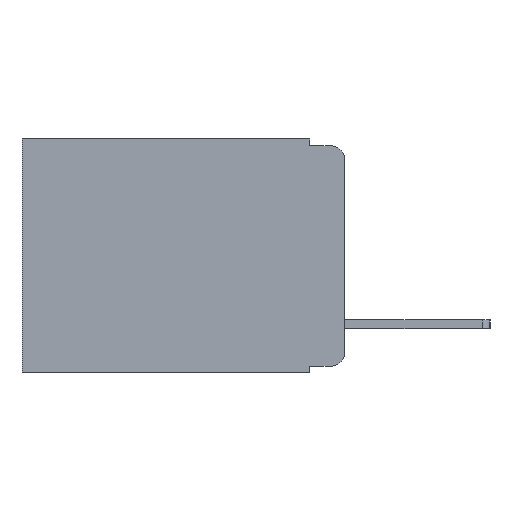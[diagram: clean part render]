
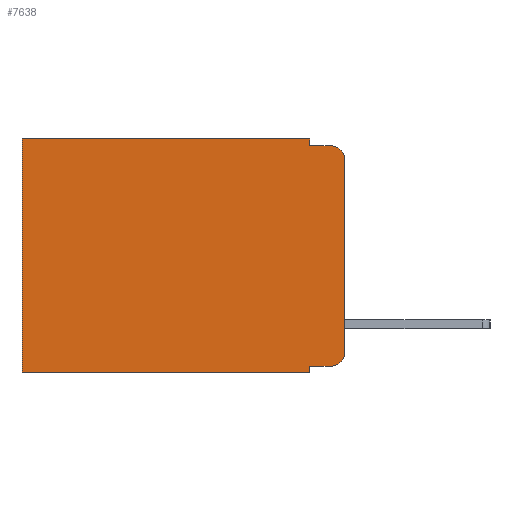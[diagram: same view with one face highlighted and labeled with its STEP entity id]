
A CAD part, left-side view. The second image highlights one B-rep face of the part: STEP entity #7638.
In plain terms, the highlighted planar face has unit normal (-1, 0, 0).
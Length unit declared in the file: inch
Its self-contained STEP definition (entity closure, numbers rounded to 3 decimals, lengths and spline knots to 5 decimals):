
#141 = LINE ( 'NONE', #13781, #4481 ) ;
#309 = DIRECTION ( 'NONE',  ( 0., 1., 0. ) ) ;
#424 = CARTESIAN_POINT ( 'NONE',  ( 0.298, 0., -0.313 ) ) ;
#872 = ORIENTED_EDGE ( 'NONE', *, *, #17467, .F. ) ;
#920 = DIRECTION ( 'NONE',  ( 0., -1., 0. ) ) ;
#971 = VERTEX_POINT ( 'NONE', #4387 ) ;
#1512 = PLANE ( 'NONE',  #5135 ) ;
#1751 = DIRECTION ( 'NONE',  ( 0., -1., 0. ) ) ;
#2066 = EDGE_CURVE ( 'NONE', #7895, #12275, #3780, .T. ) ;
#2190 = EDGE_CURVE ( 'NONE', #18293, #2368, #5958, .T. ) ;
#2220 = VECTOR ( 'NONE', #1751, 39.37008 ) ;
#2255 = CIRCLE ( 'NONE', #12514, 0.02 ) ;
#2274 = LINE ( 'NONE', #10065, #9947 ) ;
#2314 = CARTESIAN_POINT ( 'NONE',  ( 0.298, 0., -0.343 ) ) ;
#2368 = VERTEX_POINT ( 'NONE', #13191 ) ;
#3270 = EDGE_CURVE ( 'NONE', #15692, #2368, #2255, .T. ) ;
#3780 = LINE ( 'NONE', #2314, #7467 ) ;
#3826 = CARTESIAN_POINT ( 'NONE',  ( 0.298, 0.051, -0.01 ) ) ;
#4387 = CARTESIAN_POINT ( 'NONE',  ( 0.298, 0.473, 0. ) ) ;
#4481 = VECTOR ( 'NONE', #15172, 39.37008 ) ;
#4613 = DIRECTION ( 'NONE',  ( 0., 0., -1. ) ) ;
#4792 = DIRECTION ( 'NONE',  ( -1., 0., 0. ) ) ;
#4866 = EDGE_LOOP ( 'NONE', ( #11759, #19232, #8758, #872, #6126, #10129, #18152, #11023, #14870, #12000 ) ) ;
#5135 = AXIS2_PLACEMENT_3D ( 'NONE', #10736, #6286, #16503 ) ;
#5583 = VECTOR ( 'NONE', #7958, 39.37008 ) ;
#5958 = LINE ( 'NONE', #12935, #17135 ) ;
#6126 = ORIENTED_EDGE ( 'NONE', *, *, #9217, .T. ) ;
#6232 = CARTESIAN_POINT ( 'NONE',  ( 0.298, 0.051, 0. ) ) ;
#6286 = DIRECTION ( 'NONE',  ( 1., 0., 0. ) ) ;
#6385 = LINE ( 'NONE', #18024, #2220 ) ;
#6520 = CARTESIAN_POINT ( 'NONE',  ( 0.298, 0.473, 0. ) ) ;
#7467 = VECTOR ( 'NONE', #309, 39.37008 ) ;
#7604 = VERTEX_POINT ( 'NONE', #9144 ) ;
#7638 = ADVANCED_FACE ( 'NONE', ( #9001 ), #1512, .F. ) ;
#7895 = VERTEX_POINT ( 'NONE', #8508 ) ;
#7958 = DIRECTION ( 'NONE',  ( 0., 1., 0. ) ) ;
#8089 = DIRECTION ( 'NONE',  ( 0., 0., -1. ) ) ;
#8238 = DIRECTION ( 'NONE',  ( -1., 0., 0. ) ) ;
#8508 = CARTESIAN_POINT ( 'NONE',  ( 0.298, 0.051, -0.343 ) ) ;
#8758 = ORIENTED_EDGE ( 'NONE', *, *, #2190, .F. ) ;
#8840 = CIRCLE ( 'NONE', #15726, 0.02 ) ;
#9001 = FACE_OUTER_BOUND ( 'NONE', #4866, .T. ) ;
#9144 = CARTESIAN_POINT ( 'NONE',  ( 0.298, 0.051, -0.333 ) ) ;
#9217 = EDGE_CURVE ( 'NONE', #9892, #971, #16801, .T. ) ;
#9892 = VERTEX_POINT ( 'NONE', #16727 ) ;
#9947 = VECTOR ( 'NONE', #15813, 39.37008 ) ;
#10065 = CARTESIAN_POINT ( 'NONE',  ( 0.298, 0.051, 0. ) ) ;
#10077 = LINE ( 'NONE', #6520, #13530 ) ;
#10129 = ORIENTED_EDGE ( 'NONE', *, *, #16532, .T. ) ;
#10170 = CARTESIAN_POINT ( 'NONE',  ( 0.298, 0.02, -0.03 ) ) ;
#10563 = VERTEX_POINT ( 'NONE', #13039 ) ;
#10736 = CARTESIAN_POINT ( 'NONE',  ( 0.298, 0., 0. ) ) ;
#10842 = CARTESIAN_POINT ( 'NONE',  ( 0.298, 0., -0.03 ) ) ;
#10940 = VERTEX_POINT ( 'NONE', #424 ) ;
#11023 = ORIENTED_EDGE ( 'NONE', *, *, #13718, .F. ) ;
#11759 = ORIENTED_EDGE ( 'NONE', *, *, #13379, .F. ) ;
#11791 = EDGE_CURVE ( 'NONE', #10563, #10940, #8840, .T. ) ;
#12000 = ORIENTED_EDGE ( 'NONE', *, *, #11791, .T. ) ;
#12275 = VERTEX_POINT ( 'NONE', #12843 ) ;
#12514 = AXIS2_PLACEMENT_3D ( 'NONE', #10170, #4792, #4613 ) ;
#12776 = EDGE_CURVE ( 'NONE', #7604, #10563, #6385, .T. ) ;
#12843 = CARTESIAN_POINT ( 'NONE',  ( 0.298, 0.473, -0.343 ) ) ;
#12935 = CARTESIAN_POINT ( 'NONE',  ( 0.298, 0.051, -0.01 ) ) ;
#13039 = CARTESIAN_POINT ( 'NONE',  ( 0.298, 0.02, -0.333 ) ) ;
#13191 = CARTESIAN_POINT ( 'NONE',  ( 0.298, 0.02, -0.01 ) ) ;
#13379 = EDGE_CURVE ( 'NONE', #15692, #10940, #141, .T. ) ;
#13530 = VECTOR ( 'NONE', #8089, 39.37008 ) ;
#13718 = EDGE_CURVE ( 'NONE', #7604, #7895, #2274, .T. ) ;
#13733 = LINE ( 'NONE', #6232, #16575 ) ;
#13781 = CARTESIAN_POINT ( 'NONE',  ( 0.298, 0., 0. ) ) ;
#14870 = ORIENTED_EDGE ( 'NONE', *, *, #12776, .T. ) ;
#15021 = DIRECTION ( 'NONE',  ( 0., 0., -1. ) ) ;
#15172 = DIRECTION ( 'NONE',  ( 0., 0., -1. ) ) ;
#15692 = VERTEX_POINT ( 'NONE', #10842 ) ;
#15726 = AXIS2_PLACEMENT_3D ( 'NONE', #16834, #8238, #18233 ) ;
#15813 = DIRECTION ( 'NONE',  ( 0., 0., -1. ) ) ;
#16503 = DIRECTION ( 'NONE',  ( 0., 0., -1. ) ) ;
#16532 = EDGE_CURVE ( 'NONE', #971, #12275, #10077, .T. ) ;
#16568 = CARTESIAN_POINT ( 'NONE',  ( 0.298, 0., 0. ) ) ;
#16575 = VECTOR ( 'NONE', #15021, 39.37008 ) ;
#16727 = CARTESIAN_POINT ( 'NONE',  ( 0.298, 0.051, 0. ) ) ;
#16801 = LINE ( 'NONE', #16568, #5583 ) ;
#16834 = CARTESIAN_POINT ( 'NONE',  ( 0.298, 0.02, -0.313 ) ) ;
#17135 = VECTOR ( 'NONE', #920, 39.37008 ) ;
#17467 = EDGE_CURVE ( 'NONE', #9892, #18293, #13733, .T. ) ;
#18024 = CARTESIAN_POINT ( 'NONE',  ( 0.298, 0.051, -0.333 ) ) ;
#18152 = ORIENTED_EDGE ( 'NONE', *, *, #2066, .F. ) ;
#18233 = DIRECTION ( 'NONE',  ( 0., 0., -1. ) ) ;
#18293 = VERTEX_POINT ( 'NONE', #3826 ) ;
#19232 = ORIENTED_EDGE ( 'NONE', *, *, #3270, .T. ) ;
